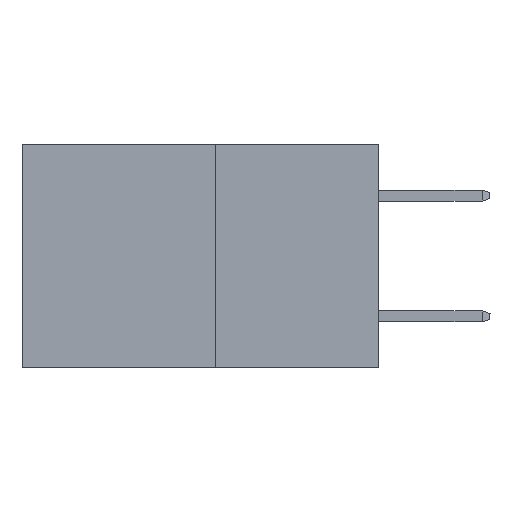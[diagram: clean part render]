
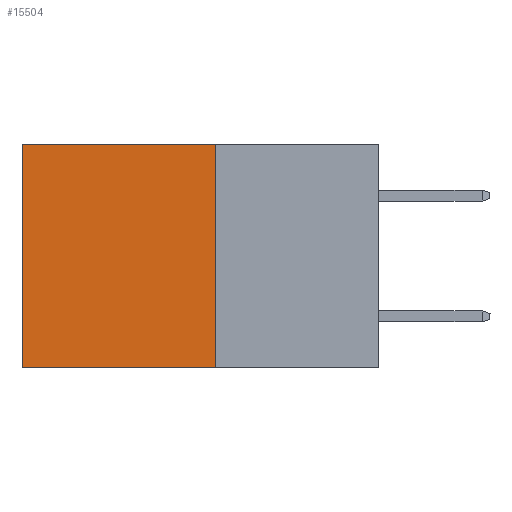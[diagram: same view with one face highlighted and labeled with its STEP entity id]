
A CAD part, left-side view. The second image highlights one B-rep face of the part: STEP entity #15504.
In plain terms, the highlighted planar face has unit normal (-1, 0, 0).
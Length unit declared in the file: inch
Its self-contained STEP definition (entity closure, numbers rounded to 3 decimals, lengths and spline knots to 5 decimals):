
#1522 = VERTEX_POINT ( 'NONE', #7728 ) ;
#1728 = PLANE ( 'NONE',  #2493 ) ;
#2493 = AXIS2_PLACEMENT_3D ( 'NONE', #3254, #4764, #14918 ) ;
#2569 = ORIENTED_EDGE ( 'NONE', *, *, #14759, .T. ) ;
#3235 = VERTEX_POINT ( 'NONE', #10646 ) ;
#3254 = CARTESIAN_POINT ( 'NONE',  ( 0.277, 0.27, -0.37 ) ) ;
#4053 = VECTOR ( 'NONE', #9366, 39.37008 ) ;
#4071 = VERTEX_POINT ( 'NONE', #16033 ) ;
#4462 = ORIENTED_EDGE ( 'NONE', *, *, #15606, .F. ) ;
#4764 = DIRECTION ( 'NONE',  ( 1., 0., 0. ) ) ;
#4935 = CARTESIAN_POINT ( 'NONE',  ( 0.277, 0.27, 0. ) ) ;
#5467 = VECTOR ( 'NONE', #6400, 39.37008 ) ;
#5763 = VECTOR ( 'NONE', #7408, 39.37008 ) ;
#6133 = VECTOR ( 'NONE', #7349, 39.37008 ) ;
#6400 = DIRECTION ( 'NONE',  ( 0., 1., 0. ) ) ;
#7349 = DIRECTION ( 'NONE',  ( 0., 0., -1. ) ) ;
#7408 = DIRECTION ( 'NONE',  ( 0., 0., -1. ) ) ;
#7415 = CARTESIAN_POINT ( 'NONE',  ( 0.277, 0.59, -0.37 ) ) ;
#7436 = CARTESIAN_POINT ( 'NONE',  ( 0.277, 0.27, -0.37 ) ) ;
#7728 = CARTESIAN_POINT ( 'NONE',  ( 0.277, 0.27, 0. ) ) ;
#8071 = EDGE_CURVE ( 'NONE', #1522, #4071, #13916, .T. ) ;
#9366 = DIRECTION ( 'NONE',  ( 0., 1., 0. ) ) ;
#10003 = CARTESIAN_POINT ( 'NONE',  ( 0.277, 0.59, 0. ) ) ;
#10646 = CARTESIAN_POINT ( 'NONE',  ( 0.277, 0.59, -0.37 ) ) ;
#10890 = LINE ( 'NONE', #18049, #4053 ) ;
#11141 = EDGE_LOOP ( 'NONE', ( #2569, #4462, #14068, #15684 ) ) ;
#13602 = FACE_OUTER_BOUND ( 'NONE', #11141, .T. ) ;
#13916 = LINE ( 'NONE', #7436, #5763 ) ;
#14068 = ORIENTED_EDGE ( 'NONE', *, *, #8071, .F. ) ;
#14759 = EDGE_CURVE ( 'NONE', #18380, #3235, #17740, .T. ) ;
#14918 = DIRECTION ( 'NONE',  ( 0., 0., -1. ) ) ;
#15504 = ADVANCED_FACE ( 'NONE', ( #13602 ), #1728, .F. ) ;
#15606 = EDGE_CURVE ( 'NONE', #4071, #3235, #10890, .T. ) ;
#15684 = ORIENTED_EDGE ( 'NONE', *, *, #17357, .T. ) ;
#16033 = CARTESIAN_POINT ( 'NONE',  ( 0.277, 0.27, -0.37 ) ) ;
#17078 = LINE ( 'NONE', #4935, #5467 ) ;
#17357 = EDGE_CURVE ( 'NONE', #1522, #18380, #17078, .T. ) ;
#17740 = LINE ( 'NONE', #7415, #6133 ) ;
#18049 = CARTESIAN_POINT ( 'NONE',  ( 0.277, 0.27, -0.37 ) ) ;
#18380 = VERTEX_POINT ( 'NONE', #10003 ) ;
